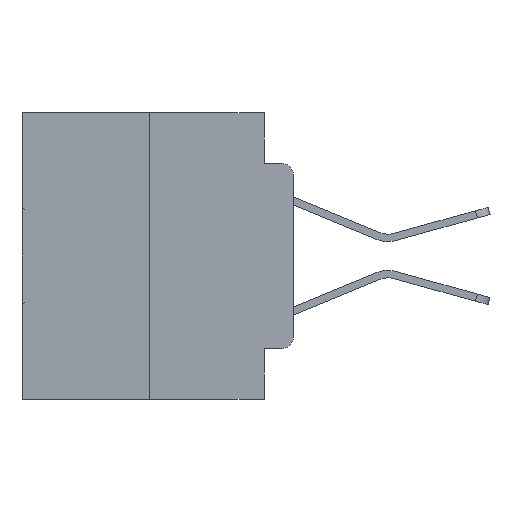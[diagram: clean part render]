
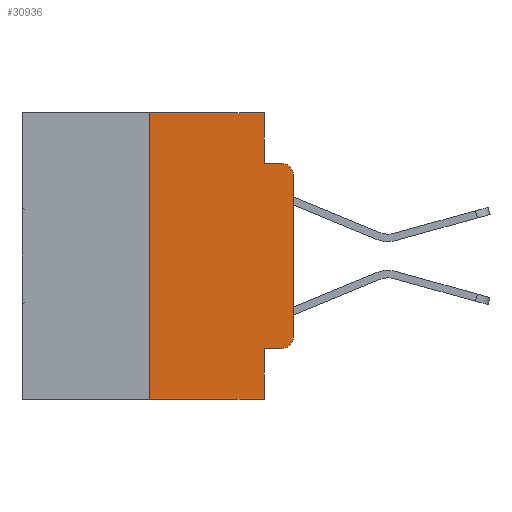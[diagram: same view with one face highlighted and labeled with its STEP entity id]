
A CAD part, left-side view. The second image highlights one B-rep face of the part: STEP entity #30936.
In plain terms, the highlighted planar face has unit normal (-1, 0, 0).
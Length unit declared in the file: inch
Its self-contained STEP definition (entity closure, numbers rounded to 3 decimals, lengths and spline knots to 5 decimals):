
#118 = LINE ( 'NONE', #1753, #920 ) ;
#240 = ORIENTED_EDGE ( 'NONE', *, *, #11678, .T. ) ;
#838 = ORIENTED_EDGE ( 'NONE', *, *, #845, .T. ) ;
#845 = EDGE_CURVE ( 'NONE', #5519, #19512, #17204, .T. ) ;
#920 = VECTOR ( 'NONE', #4265, 39.37008 ) ;
#1367 = DIRECTION ( 'NONE',  ( 0., 0., 1. ) ) ;
#1475 = ORIENTED_EDGE ( 'NONE', *, *, #30295, .F. ) ;
#1753 = CARTESIAN_POINT ( 'NONE',  ( 0., 0.473, -0.5 ) ) ;
#1790 = ORIENTED_EDGE ( 'NONE', *, *, #7670, .F. ) ;
#1800 = ORIENTED_EDGE ( 'NONE', *, *, #10111, .T. ) ;
#1988 = VERTEX_POINT ( 'NONE', #19401 ) ;
#2216 = CARTESIAN_POINT ( 'NONE',  ( 0., 0.25, 0. ) ) ;
#2796 = VERTEX_POINT ( 'NONE', #8702 ) ;
#2952 = VERTEX_POINT ( 'NONE', #23793 ) ;
#2993 = ORIENTED_EDGE ( 'NONE', *, *, #11488, .T. ) ;
#3032 = AXIS2_PLACEMENT_3D ( 'NONE', #12051, #28798, #14479 ) ;
#3181 = AXIS2_PLACEMENT_3D ( 'NONE', #4573, #31032, #16834 ) ;
#3198 = VECTOR ( 'NONE', #11355, 39.37008 ) ;
#3549 = EDGE_CURVE ( 'NONE', #7182, #1988, #22603, .T. ) ;
#3863 = LINE ( 'NONE', #6259, #28749 ) ;
#3896 = CARTESIAN_POINT ( 'NONE',  ( 0., 0.051, -0.4115 ) ) ;
#4204 = VECTOR ( 'NONE', #30698, 39.37008 ) ;
#4265 = DIRECTION ( 'NONE',  ( 0., -1., 0. ) ) ;
#4427 = ORIENTED_EDGE ( 'NONE', *, *, #16995, .T. ) ;
#4573 = CARTESIAN_POINT ( 'NONE',  ( 0., 0.473, 0. ) ) ;
#5271 = ORIENTED_EDGE ( 'NONE', *, *, #15998, .F. ) ;
#5290 = VECTOR ( 'NONE', #30343, 39.37008 ) ;
#5519 = VERTEX_POINT ( 'NONE', #3896 ) ;
#6259 = CARTESIAN_POINT ( 'NONE',  ( 0., 0., 0. ) ) ;
#6416 = DIRECTION ( 'NONE',  ( -1., 0., 0. ) ) ;
#6938 = AXIS2_PLACEMENT_3D ( 'NONE', #20945, #6416, #23363 ) ;
#6966 = DIRECTION ( 'NONE',  ( 0., -1., 0. ) ) ;
#7119 = CARTESIAN_POINT ( 'NONE',  ( 0., 0.051, -0.5 ) ) ;
#7182 = VERTEX_POINT ( 'NONE', #12521 ) ;
#7670 = EDGE_CURVE ( 'NONE', #29988, #2796, #27226, .T. ) ;
#7686 = CARTESIAN_POINT ( 'NONE',  ( 0., 0.25, -0.5 ) ) ;
#8702 = CARTESIAN_POINT ( 'NONE',  ( 0., 0.25, 0. ) ) ;
#9548 = VECTOR ( 'NONE', #19323, 39.37008 ) ;
#10111 = EDGE_CURVE ( 'NONE', #29988, #25028, #118, .T. ) ;
#10465 = VERTEX_POINT ( 'NONE', #21758 ) ;
#11152 = CARTESIAN_POINT ( 'NONE',  ( 0., 0.051, 0. ) ) ;
#11355 = DIRECTION ( 'NONE',  ( 0., 0., -1. ) ) ;
#11488 = EDGE_CURVE ( 'NONE', #2952, #14423, #29952, .T. ) ;
#11678 = EDGE_CURVE ( 'NONE', #19512, #10465, #31048, .T. ) ;
#12051 = CARTESIAN_POINT ( 'NONE',  ( 0., 0.02, -0.3915 ) ) ;
#12479 = CARTESIAN_POINT ( 'NONE',  ( 0., 0.473, 0. ) ) ;
#12521 = CARTESIAN_POINT ( 'NONE',  ( 0., 0.051, 0. ) ) ;
#12719 = VECTOR ( 'NONE', #14923, 39.37008 ) ;
#13425 = ORIENTED_EDGE ( 'NONE', *, *, #3549, .F. ) ;
#13629 = CARTESIAN_POINT ( 'NONE',  ( 0., 0.051, 0. ) ) ;
#14423 = VERTEX_POINT ( 'NONE', #25557 ) ;
#14479 = DIRECTION ( 'NONE',  ( 0., 0., -1. ) ) ;
#14923 = DIRECTION ( 'NONE',  ( 0., -1., 0. ) ) ;
#15025 = EDGE_LOOP ( 'NONE', ( #4427, #2993, #17793, #13425, #5271, #1790, #1800, #1475, #838, #240 ) ) ;
#15998 = EDGE_CURVE ( 'NONE', #2796, #7182, #19205, .T. ) ;
#16082 = LINE ( 'NONE', #23894, #20225 ) ;
#16834 = DIRECTION ( 'NONE',  ( 0., 0., -1. ) ) ;
#16995 = EDGE_CURVE ( 'NONE', #10465, #2952, #3863, .T. ) ;
#17082 = FACE_OUTER_BOUND ( 'NONE', #15025, .T. ) ;
#17204 = LINE ( 'NONE', #22910, #4204 ) ;
#17793 = ORIENTED_EDGE ( 'NONE', *, *, #24413, .F. ) ;
#19205 = LINE ( 'NONE', #12479, #12719 ) ;
#19323 = DIRECTION ( 'NONE',  ( 0., 0., 1. ) ) ;
#19401 = CARTESIAN_POINT ( 'NONE',  ( 0., 0.051, -0.0885 ) ) ;
#19512 = VERTEX_POINT ( 'NONE', #26067 ) ;
#20225 = VECTOR ( 'NONE', #6966, 39.37008 ) ;
#20945 = CARTESIAN_POINT ( 'NONE',  ( 0., 0.02, -0.1085 ) ) ;
#21758 = CARTESIAN_POINT ( 'NONE',  ( 0., 0., -0.3915 ) ) ;
#22603 = LINE ( 'NONE', #11152, #3198 ) ;
#22910 = CARTESIAN_POINT ( 'NONE',  ( 0., 0.051, -0.4115 ) ) ;
#23363 = DIRECTION ( 'NONE',  ( 0., 0., -1. ) ) ;
#23793 = CARTESIAN_POINT ( 'NONE',  ( 0., 0., -0.1085 ) ) ;
#23847 = LINE ( 'NONE', #13629, #5290 ) ;
#23894 = CARTESIAN_POINT ( 'NONE',  ( 0., 0.051, -0.0885 ) ) ;
#24413 = EDGE_CURVE ( 'NONE', #1988, #14423, #16082, .T. ) ;
#25028 = VERTEX_POINT ( 'NONE', #7119 ) ;
#25557 = CARTESIAN_POINT ( 'NONE',  ( 0., 0.02, -0.0885 ) ) ;
#26067 = CARTESIAN_POINT ( 'NONE',  ( 0., 0.02, -0.4115 ) ) ;
#27226 = LINE ( 'NONE', #2216, #9548 ) ;
#28664 = PLANE ( 'NONE',  #3181 ) ;
#28749 = VECTOR ( 'NONE', #1367, 39.37008 ) ;
#28798 = DIRECTION ( 'NONE',  ( -1., 0., 0. ) ) ;
#29952 = CIRCLE ( 'NONE', #6938, 0.02 ) ;
#29988 = VERTEX_POINT ( 'NONE', #7686 ) ;
#30295 = EDGE_CURVE ( 'NONE', #5519, #25028, #23847, .T. ) ;
#30343 = DIRECTION ( 'NONE',  ( 0., 0., -1. ) ) ;
#30698 = DIRECTION ( 'NONE',  ( 0., -1., 0. ) ) ;
#30936 = ADVANCED_FACE ( 'NONE', ( #17082 ), #28664, .F. ) ;
#31032 = DIRECTION ( 'NONE',  ( 1., 0., 0. ) ) ;
#31048 = CIRCLE ( 'NONE', #3032, 0.02 ) ;
